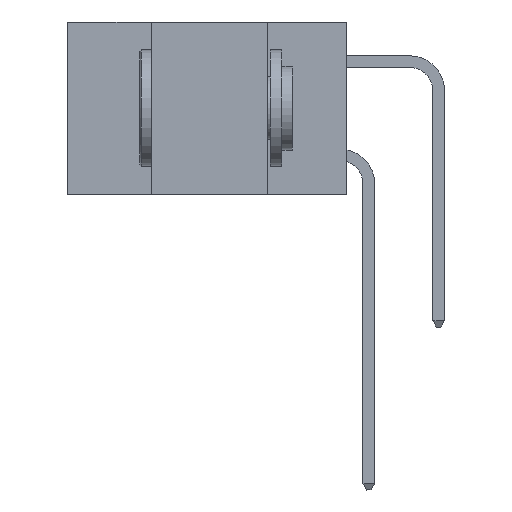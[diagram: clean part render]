
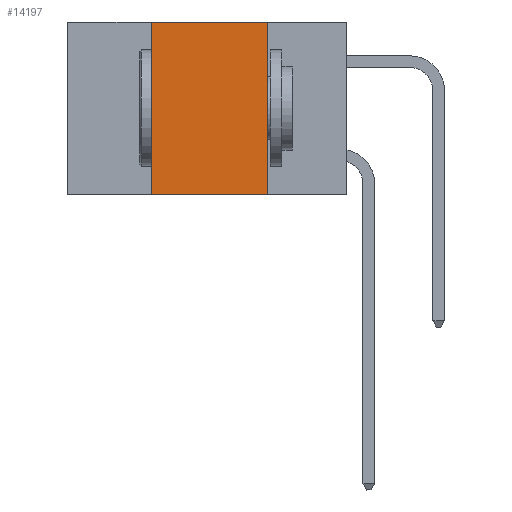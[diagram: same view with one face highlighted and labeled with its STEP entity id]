
A CAD part, left-side view. The second image highlights one B-rep face of the part: STEP entity #14197.
In plain terms, the highlighted planar face has unit normal (-1, 0, 0).
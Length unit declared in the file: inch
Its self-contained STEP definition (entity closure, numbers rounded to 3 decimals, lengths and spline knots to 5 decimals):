
#486 = VECTOR ( 'NONE', #12520, 39.37008 ) ;
#2379 = LINE ( 'NONE', #26780, #7970 ) ;
#2873 = DIRECTION ( 'NONE',  ( 0., -1., 0. ) ) ;
#4033 = VERTEX_POINT ( 'NONE', #26941 ) ;
#4728 = ORIENTED_EDGE ( 'NONE', *, *, #10927, .F. ) ;
#4825 = DIRECTION ( 'NONE',  ( 1., 0., 0. ) ) ;
#7179 = FACE_OUTER_BOUND ( 'NONE', #22314, .T. ) ;
#7970 = VECTOR ( 'NONE', #38329, 39.37008 ) ;
#8566 = VECTOR ( 'NONE', #29896, 39.37008 ) ;
#8914 = VERTEX_POINT ( 'NONE', #13977 ) ;
#10927 = EDGE_CURVE ( 'NONE', #8914, #33618, #19885, .T. ) ;
#11788 = LINE ( 'NONE', #20474, #8566 ) ;
#11805 = CARTESIAN_POINT ( 'NONE',  ( 0., 0.42, -0.37 ) ) ;
#12082 = CARTESIAN_POINT ( 'NONE',  ( 0., 0.6, 0. ) ) ;
#12520 = DIRECTION ( 'NONE',  ( 0., 0., 1. ) ) ;
#13977 = CARTESIAN_POINT ( 'NONE',  ( 0., 0.42, 0. ) ) ;
#14197 = ADVANCED_FACE ( 'NONE', ( #7179 ), #19780, .F. ) ;
#14274 = VECTOR ( 'NONE', #2873, 39.37008 ) ;
#14548 = ORIENTED_EDGE ( 'NONE', *, *, #35225, .F. ) ;
#15145 = CARTESIAN_POINT ( 'NONE',  ( 0., 0.42, 0. ) ) ;
#19074 = LINE ( 'NONE', #15145, #486 ) ;
#19780 = PLANE ( 'NONE',  #27657 ) ;
#19885 = LINE ( 'NONE', #12082, #14274 ) ;
#20474 = CARTESIAN_POINT ( 'NONE',  ( 0., 0.6, -0.37 ) ) ;
#22314 = EDGE_LOOP ( 'NONE', ( #33711, #4728, #14548, #30380 ) ) ;
#26538 = EDGE_CURVE ( 'NONE', #33618, #4033, #2379, .T. ) ;
#26780 = CARTESIAN_POINT ( 'NONE',  ( 0., 0.17, 0. ) ) ;
#26941 = CARTESIAN_POINT ( 'NONE',  ( 0., 0.17, -0.37 ) ) ;
#27657 = AXIS2_PLACEMENT_3D ( 'NONE', #38001, #4825, #29086 ) ;
#29086 = DIRECTION ( 'NONE',  ( 0., 0., -1. ) ) ;
#29896 = DIRECTION ( 'NONE',  ( 0., -1., 0. ) ) ;
#30380 = ORIENTED_EDGE ( 'NONE', *, *, #33257, .T. ) ;
#33257 = EDGE_CURVE ( 'NONE', #34445, #4033, #11788, .T. ) ;
#33618 = VERTEX_POINT ( 'NONE', #37073 ) ;
#33711 = ORIENTED_EDGE ( 'NONE', *, *, #26538, .F. ) ;
#34445 = VERTEX_POINT ( 'NONE', #11805 ) ;
#35225 = EDGE_CURVE ( 'NONE', #34445, #8914, #19074, .T. ) ;
#37073 = CARTESIAN_POINT ( 'NONE',  ( 0., 0.17, 0. ) ) ;
#38001 = CARTESIAN_POINT ( 'NONE',  ( 0., 0.6, 0. ) ) ;
#38329 = DIRECTION ( 'NONE',  ( 0., 0., -1. ) ) ;
